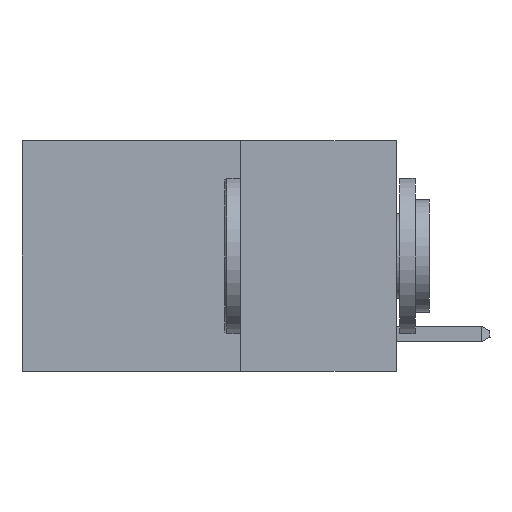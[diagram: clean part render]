
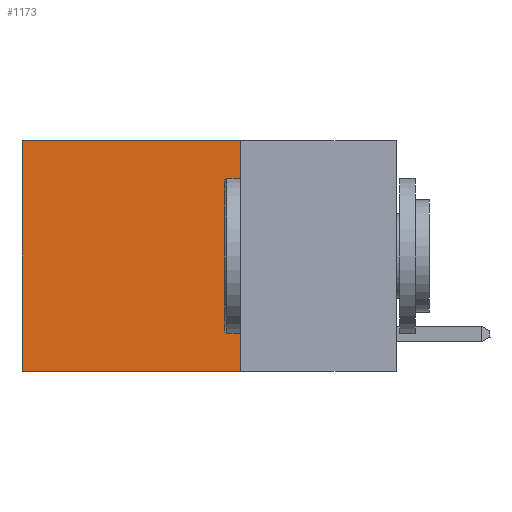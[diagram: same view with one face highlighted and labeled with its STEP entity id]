
A CAD part, left-side view. The second image highlights one B-rep face of the part: STEP entity #1173.
In plain terms, the highlighted planar face has unit normal (-1, 0, 0).
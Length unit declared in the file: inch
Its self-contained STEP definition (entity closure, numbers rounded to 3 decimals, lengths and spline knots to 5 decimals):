
#142 = CARTESIAN_POINT ( 'NONE',  ( 0.2625, 0.25, -0.37 ) ) ;
#1173 = ADVANCED_FACE ( 'NONE', ( #22335 ), #6822, .F. ) ;
#1629 = CARTESIAN_POINT ( 'NONE',  ( 0.2625, 0.6, -0.37 ) ) ;
#2878 = EDGE_CURVE ( 'NONE', #5663, #5595, #15791, .T. ) ;
#3453 = DIRECTION ( 'NONE',  ( 0., 0., -1. ) ) ;
#4224 = CARTESIAN_POINT ( 'NONE',  ( 0.2625, 0.25, 0. ) ) ;
#5134 = VERTEX_POINT ( 'NONE', #1629 ) ;
#5274 = DIRECTION ( 'NONE',  ( 1., 0., 0. ) ) ;
#5595 = VERTEX_POINT ( 'NONE', #22604 ) ;
#5663 = VERTEX_POINT ( 'NONE', #25052 ) ;
#6822 = PLANE ( 'NONE',  #7489 ) ;
#6839 = CARTESIAN_POINT ( 'NONE',  ( 0.2625, 0.25, 0. ) ) ;
#6985 = EDGE_CURVE ( 'NONE', #5663, #10382, #24946, .T. ) ;
#7046 = EDGE_LOOP ( 'NONE', ( #20146, #9188, #7375, #20845 ) ) ;
#7375 = ORIENTED_EDGE ( 'NONE', *, *, #2878, .F. ) ;
#7489 = AXIS2_PLACEMENT_3D ( 'NONE', #18928, #5274, #3453 ) ;
#7556 = VECTOR ( 'NONE', #8217, 39.37008 ) ;
#8217 = DIRECTION ( 'NONE',  ( 0., 0., -1. ) ) ;
#9004 = LINE ( 'NONE', #24886, #25108 ) ;
#9086 = VECTOR ( 'NONE', #17568, 39.37008 ) ;
#9188 = ORIENTED_EDGE ( 'NONE', *, *, #10245, .F. ) ;
#10245 = EDGE_CURVE ( 'NONE', #5595, #5134, #23705, .T. ) ;
#10382 = VERTEX_POINT ( 'NONE', #12789 ) ;
#12789 = CARTESIAN_POINT ( 'NONE',  ( 0.2625, 0.6, 0. ) ) ;
#15791 = LINE ( 'NONE', #4224, #7556 ) ;
#17568 = DIRECTION ( 'NONE',  ( 0., 1., 0. ) ) ;
#18063 = VECTOR ( 'NONE', #21013, 39.37008 ) ;
#18928 = CARTESIAN_POINT ( 'NONE',  ( 0.2625, 0.25, 0. ) ) ;
#20146 = ORIENTED_EDGE ( 'NONE', *, *, #20218, .T. ) ;
#20218 = EDGE_CURVE ( 'NONE', #10382, #5134, #9004, .T. ) ;
#20845 = ORIENTED_EDGE ( 'NONE', *, *, #6985, .T. ) ;
#21013 = DIRECTION ( 'NONE',  ( 0., 1., 0. ) ) ;
#22335 = FACE_OUTER_BOUND ( 'NONE', #7046, .T. ) ;
#22604 = CARTESIAN_POINT ( 'NONE',  ( 0.2625, 0.25, -0.37 ) ) ;
#22931 = DIRECTION ( 'NONE',  ( 0., 0., -1. ) ) ;
#23705 = LINE ( 'NONE', #142, #9086 ) ;
#24886 = CARTESIAN_POINT ( 'NONE',  ( 0.2625, 0.6, 0. ) ) ;
#24946 = LINE ( 'NONE', #6839, #18063 ) ;
#25052 = CARTESIAN_POINT ( 'NONE',  ( 0.2625, 0.25, 0. ) ) ;
#25108 = VECTOR ( 'NONE', #22931, 39.37008 ) ;
